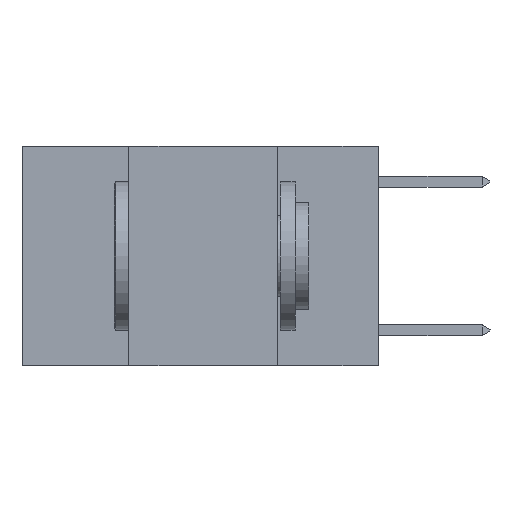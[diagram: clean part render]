
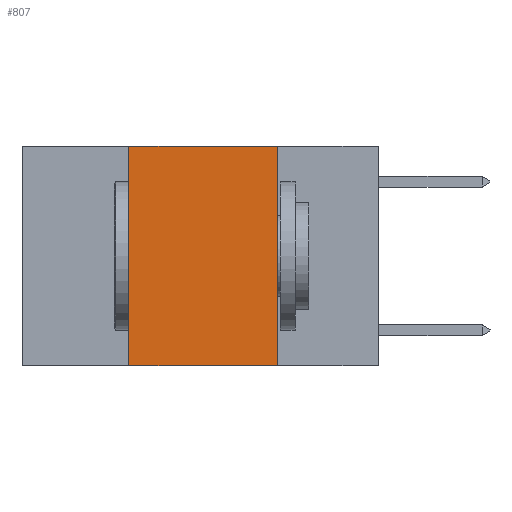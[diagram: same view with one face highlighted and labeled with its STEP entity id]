
A CAD part, left-side view. The second image highlights one B-rep face of the part: STEP entity #807.
In plain terms, the highlighted planar face has unit normal (-1, 0, 0).
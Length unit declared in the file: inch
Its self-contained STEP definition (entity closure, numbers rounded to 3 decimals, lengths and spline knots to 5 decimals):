
#191 = CARTESIAN_POINT ( 'NONE',  ( 0., 0.42, 0. ) ) ;
#731 = EDGE_CURVE ( 'NONE', #2126, #2396, #9519, .T. ) ;
#807 = ADVANCED_FACE ( 'NONE', ( #10409 ), #6588, .F. ) ;
#811 = ORIENTED_EDGE ( 'NONE', *, *, #7128, .F. ) ;
#1100 = DIRECTION ( 'NONE',  ( 0., -1., 0. ) ) ;
#1256 = CARTESIAN_POINT ( 'NONE',  ( 0., 0.17, -0.37 ) ) ;
#1516 = LINE ( 'NONE', #6354, #10211 ) ;
#1784 = ORIENTED_EDGE ( 'NONE', *, *, #731, .F. ) ;
#2126 = VERTEX_POINT ( 'NONE', #5472 ) ;
#2148 = EDGE_LOOP ( 'NONE', ( #8856, #811, #1784, #8577 ) ) ;
#2396 = VERTEX_POINT ( 'NONE', #5099 ) ;
#2679 = AXIS2_PLACEMENT_3D ( 'NONE', #6766, #7044, #6969 ) ;
#2920 = LINE ( 'NONE', #6320, #7173 ) ;
#3190 = VECTOR ( 'NONE', #5934, 39.37008 ) ;
#3245 = EDGE_CURVE ( 'NONE', #5038, #6419, #6987, .T. ) ;
#4110 = DIRECTION ( 'NONE',  ( 0., 0., -1. ) ) ;
#5038 = VERTEX_POINT ( 'NONE', #8044 ) ;
#5099 = CARTESIAN_POINT ( 'NONE',  ( 0., 0.42, 0. ) ) ;
#5472 = CARTESIAN_POINT ( 'NONE',  ( 0., 0.42, -0.37 ) ) ;
#5934 = DIRECTION ( 'NONE',  ( 0., 0., 1. ) ) ;
#6320 = CARTESIAN_POINT ( 'NONE',  ( 0., 0.6, 0. ) ) ;
#6354 = CARTESIAN_POINT ( 'NONE',  ( 0., 0.6, -0.37 ) ) ;
#6419 = VERTEX_POINT ( 'NONE', #1256 ) ;
#6588 = PLANE ( 'NONE',  #2679 ) ;
#6766 = CARTESIAN_POINT ( 'NONE',  ( 0., 0.6, 0. ) ) ;
#6969 = DIRECTION ( 'NONE',  ( 0., 0., -1. ) ) ;
#6987 = LINE ( 'NONE', #9820, #10996 ) ;
#7044 = DIRECTION ( 'NONE',  ( 1., 0., 0. ) ) ;
#7128 = EDGE_CURVE ( 'NONE', #2396, #5038, #2920, .T. ) ;
#7140 = DIRECTION ( 'NONE',  ( 0., -1., 0. ) ) ;
#7173 = VECTOR ( 'NONE', #7140, 39.37008 ) ;
#8044 = CARTESIAN_POINT ( 'NONE',  ( 0., 0.17, 0. ) ) ;
#8577 = ORIENTED_EDGE ( 'NONE', *, *, #10167, .T. ) ;
#8856 = ORIENTED_EDGE ( 'NONE', *, *, #3245, .F. ) ;
#9519 = LINE ( 'NONE', #191, #3190 ) ;
#9820 = CARTESIAN_POINT ( 'NONE',  ( 0., 0.17, 0. ) ) ;
#10167 = EDGE_CURVE ( 'NONE', #2126, #6419, #1516, .T. ) ;
#10211 = VECTOR ( 'NONE', #1100, 39.37008 ) ;
#10409 = FACE_OUTER_BOUND ( 'NONE', #2148, .T. ) ;
#10996 = VECTOR ( 'NONE', #4110, 39.37008 ) ;
